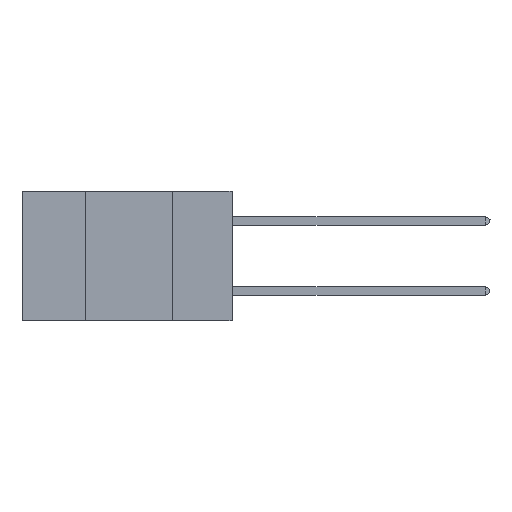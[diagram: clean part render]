
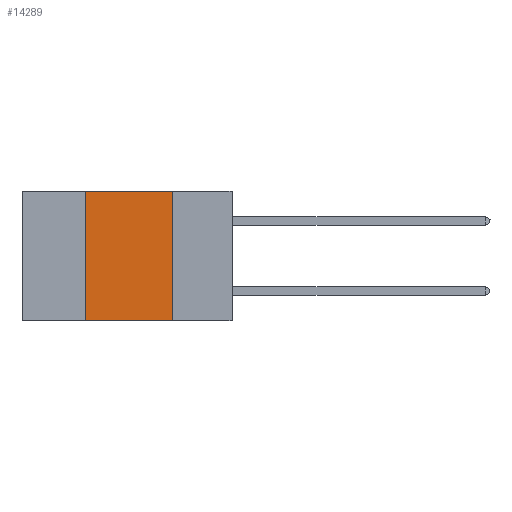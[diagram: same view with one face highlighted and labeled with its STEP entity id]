
A CAD part, left-side view. The second image highlights one B-rep face of the part: STEP entity #14289.
In plain terms, the highlighted planar face has unit normal (-1, 0, 0).
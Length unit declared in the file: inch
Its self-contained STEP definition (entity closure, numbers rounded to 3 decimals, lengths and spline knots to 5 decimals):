
#1311 = DIRECTION ( 'NONE',  ( 1., 0., 0. ) ) ;
#2087 = ORIENTED_EDGE ( 'NONE', *, *, #9458, .F. ) ;
#2398 = CARTESIAN_POINT ( 'NONE',  ( 0., 0.42, 0. ) ) ;
#3213 = LINE ( 'NONE', #2398, #9519 ) ;
#4405 = LINE ( 'NONE', #29834, #37380 ) ;
#5317 = DIRECTION ( 'NONE',  ( 0., 0., -1. ) ) ;
#5875 = VERTEX_POINT ( 'NONE', #25185 ) ;
#8126 = DIRECTION ( 'NONE',  ( 0., -1., 0. ) ) ;
#8578 = CARTESIAN_POINT ( 'NONE',  ( 0., 0.6, 0. ) ) ;
#9458 = EDGE_CURVE ( 'NONE', #19355, #37412, #17169, .T. ) ;
#9519 = VECTOR ( 'NONE', #37225, 39.37008 ) ;
#14289 = ADVANCED_FACE ( 'NONE', ( #15730 ), #20194, .F. ) ;
#15730 = FACE_OUTER_BOUND ( 'NONE', #36028, .T. ) ;
#16429 = DIRECTION ( 'NONE',  ( 0., -1., 0. ) ) ;
#17169 = LINE ( 'NONE', #8578, #27335 ) ;
#17626 = CARTESIAN_POINT ( 'NONE',  ( 0., 0.42, -0.37 ) ) ;
#19355 = VERTEX_POINT ( 'NONE', #40162 ) ;
#19929 = CARTESIAN_POINT ( 'NONE',  ( 0., 0.6, 0. ) ) ;
#19932 = CARTESIAN_POINT ( 'NONE',  ( 0., 0.17, 0. ) ) ;
#20194 = PLANE ( 'NONE',  #21857 ) ;
#21857 = AXIS2_PLACEMENT_3D ( 'NONE', #19929, #1311, #23154 ) ;
#22853 = LINE ( 'NONE', #31590, #29593 ) ;
#23154 = DIRECTION ( 'NONE',  ( 0., 0., -1. ) ) ;
#25185 = CARTESIAN_POINT ( 'NONE',  ( 0., 0.17, -0.37 ) ) ;
#27335 = VECTOR ( 'NONE', #8126, 39.37008 ) ;
#27628 = EDGE_CURVE ( 'NONE', #32118, #19355, #3213, .T. ) ;
#28193 = EDGE_CURVE ( 'NONE', #32118, #5875, #22853, .T. ) ;
#29593 = VECTOR ( 'NONE', #16429, 39.37008 ) ;
#29834 = CARTESIAN_POINT ( 'NONE',  ( 0., 0.17, 0. ) ) ;
#31375 = ORIENTED_EDGE ( 'NONE', *, *, #27628, .F. ) ;
#31590 = CARTESIAN_POINT ( 'NONE',  ( 0., 0.6, -0.37 ) ) ;
#32118 = VERTEX_POINT ( 'NONE', #17626 ) ;
#34234 = ORIENTED_EDGE ( 'NONE', *, *, #28193, .T. ) ;
#34384 = ORIENTED_EDGE ( 'NONE', *, *, #34653, .F. ) ;
#34653 = EDGE_CURVE ( 'NONE', #37412, #5875, #4405, .T. ) ;
#36028 = EDGE_LOOP ( 'NONE', ( #34384, #2087, #31375, #34234 ) ) ;
#37225 = DIRECTION ( 'NONE',  ( 0., 0., 1. ) ) ;
#37380 = VECTOR ( 'NONE', #5317, 39.37008 ) ;
#37412 = VERTEX_POINT ( 'NONE', #19932 ) ;
#40162 = CARTESIAN_POINT ( 'NONE',  ( 0., 0.42, 0. ) ) ;
